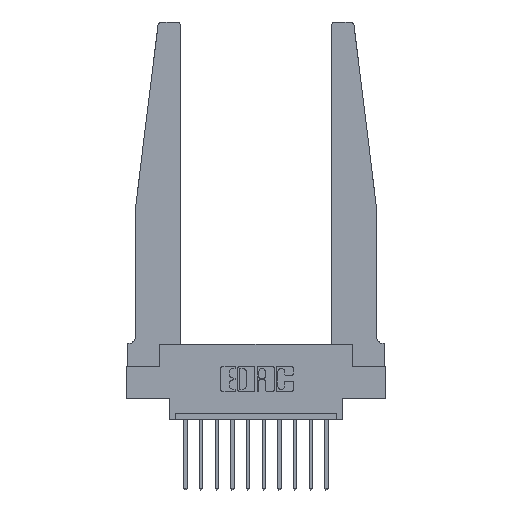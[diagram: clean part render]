
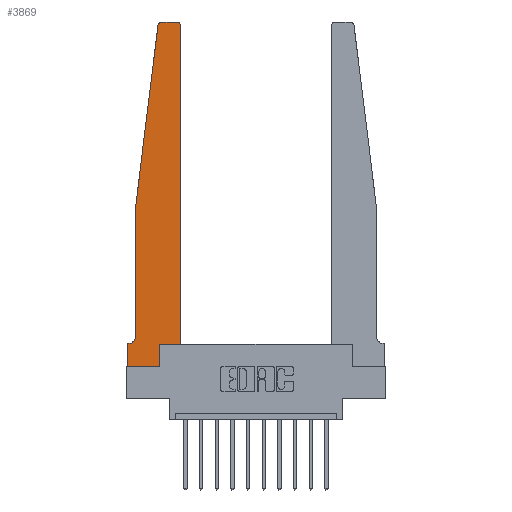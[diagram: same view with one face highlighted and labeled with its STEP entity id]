
A CAD part, top view. The second image highlights one B-rep face of the part: STEP entity #3869.
In plain terms, the highlighted planar face has unit normal (0, 0, 1).
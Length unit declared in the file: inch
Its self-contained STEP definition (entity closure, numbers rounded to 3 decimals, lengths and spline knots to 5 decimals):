
#71 = VECTOR ( 'NONE', #14322, 39.37008 ) ;
#1012 = VECTOR ( 'NONE', #14533, 39.37008 ) ;
#1158 = VERTEX_POINT ( 'NONE', #6319 ) ;
#1197 = ORIENTED_EDGE ( 'NONE', *, *, #5497, .T. ) ;
#1796 = CIRCLE ( 'NONE', #9764, 0.05 ) ;
#1976 = CARTESIAN_POINT ( 'NONE',  ( 0.2605, 0., 0.37 ) ) ;
#2045 = ORIENTED_EDGE ( 'NONE', *, *, #12021, .T. ) ;
#2255 = ORIENTED_EDGE ( 'NONE', *, *, #13639, .T. ) ;
#2366 = VERTEX_POINT ( 'NONE', #6105 ) ;
#2495 = VECTOR ( 'NONE', #3002, 39.37008 ) ;
#2706 = DIRECTION ( 'NONE',  ( 0., 0., 1. ) ) ;
#2829 = CARTESIAN_POINT ( 'NONE',  ( 0.25, 2.75, 0.37 ) ) ;
#2852 = CARTESIAN_POINT ( 'NONE',  ( 0.24675, 2.72367, 0.37 ) ) ;
#2860 = CARTESIAN_POINT ( 'NONE',  ( 0., 0., 0.37 ) ) ;
#2919 = EDGE_CURVE ( 'NONE', #6110, #9453, #13456, .T. ) ;
#2981 = CARTESIAN_POINT ( 'NONE',  ( 0.065, 1.25, 0.37 ) ) ;
#3002 = DIRECTION ( 'NONE',  ( 1., 0., 0. ) ) ;
#3043 = VECTOR ( 'NONE', #7891, 39.37008 ) ;
#3121 = FACE_OUTER_BOUND ( 'NONE', #15692, .T. ) ;
#3164 = CARTESIAN_POINT ( 'NONE',  ( 0.425, 0.18, 0.37 ) ) ;
#3613 = CARTESIAN_POINT ( 'NONE',  ( 0.27653, 2.75, 0.37 ) ) ;
#3869 = ADVANCED_FACE ( 'NONE', ( #3121 ), #15094, .T. ) ;
#4030 = DIRECTION ( 'NONE',  ( 0., 0., -1. ) ) ;
#4050 = EDGE_CURVE ( 'NONE', #10909, #1158, #6013, .T. ) ;
#4163 = DIRECTION ( 'NONE',  ( 1., 0., 0. ) ) ;
#4187 = LINE ( 'NONE', #2981, #3043 ) ;
#4429 = CARTESIAN_POINT ( 'NONE',  ( 0.425, 0.18, 0.37 ) ) ;
#4906 = ORIENTED_EDGE ( 'NONE', *, *, #12442, .T. ) ;
#4999 = CARTESIAN_POINT ( 'NONE',  ( 0.015, 0.2375, 0.37 ) ) ;
#5060 = VECTOR ( 'NONE', #11348, 39.37008 ) ;
#5497 = EDGE_CURVE ( 'NONE', #6813, #14636, #7718, .T. ) ;
#5702 = CARTESIAN_POINT ( 'NONE',  ( 0.065, 0.1875, 0.37 ) ) ;
#5705 = ORIENTED_EDGE ( 'NONE', *, *, #7953, .T. ) ;
#6013 = LINE ( 'NONE', #15486, #15292 ) ;
#6105 = CARTESIAN_POINT ( 'NONE',  ( 0.2605, 0.18, 0.37 ) ) ;
#6110 = VERTEX_POINT ( 'NONE', #8705 ) ;
#6305 = EDGE_CURVE ( 'NONE', #11668, #6110, #15426, .T. ) ;
#6319 = CARTESIAN_POINT ( 'NONE',  ( 0.065, 1.25, 0.37 ) ) ;
#6813 = VERTEX_POINT ( 'NONE', #2860 ) ;
#7058 = ORIENTED_EDGE ( 'NONE', *, *, #4050, .T. ) ;
#7499 = EDGE_CURVE ( 'NONE', #1158, #8719, #4187, .T. ) ;
#7537 = ORIENTED_EDGE ( 'NONE', *, *, #8444, .T. ) ;
#7700 = VERTEX_POINT ( 'NONE', #3613 ) ;
#7718 = LINE ( 'NONE', #14945, #5060 ) ;
#7891 = DIRECTION ( 'NONE',  ( 0., -1., 0. ) ) ;
#7933 = CIRCLE ( 'NONE', #11028, 0.03 ) ;
#7953 = EDGE_CURVE ( 'NONE', #9006, #15845, #10551, .T. ) ;
#8186 = CARTESIAN_POINT ( 'NONE',  ( 0.425, 0.18, 0.37 ) ) ;
#8212 = CARTESIAN_POINT ( 'NONE',  ( 0.065, 0.2375, 0.37 ) ) ;
#8260 = DIRECTION ( 'NONE',  ( -0.122, -0.992, 0. ) ) ;
#8275 = CARTESIAN_POINT ( 'NONE',  ( 0., 0., 0.37 ) ) ;
#8371 = LINE ( 'NONE', #15761, #12905 ) ;
#8444 = EDGE_CURVE ( 'NONE', #8719, #9006, #1796, .T. ) ;
#8705 = CARTESIAN_POINT ( 'NONE',  ( 0.425, 2.72, 0.37 ) ) ;
#8719 = VERTEX_POINT ( 'NONE', #8212 ) ;
#8927 = LINE ( 'NONE', #2829, #71 ) ;
#8940 = DIRECTION ( 'NONE',  ( -1., 0., 0. ) ) ;
#8989 = CARTESIAN_POINT ( 'NONE',  ( 0.395, 2.75, 0.37 ) ) ;
#9006 = VERTEX_POINT ( 'NONE', #14004 ) ;
#9335 = DIRECTION ( 'NONE',  ( 0., 1., 0. ) ) ;
#9358 = LINE ( 'NONE', #3164, #2495 ) ;
#9453 = VERTEX_POINT ( 'NONE', #8989 ) ;
#9570 = VECTOR ( 'NONE', #15505, 39.37008 ) ;
#9764 = AXIS2_PLACEMENT_3D ( 'NONE', #4999, #4030, #8940 ) ;
#10368 = DIRECTION ( 'NONE',  ( 0., 0., 1. ) ) ;
#10551 = LINE ( 'NONE', #5702, #1012 ) ;
#10583 = DIRECTION ( 'NONE',  ( 0., 1., 0. ) ) ;
#10752 = ORIENTED_EDGE ( 'NONE', *, *, #2919, .T. ) ;
#10830 = ORIENTED_EDGE ( 'NONE', *, *, #11289, .T. ) ;
#10873 = DIRECTION ( 'NONE',  ( 1., 0., 0. ) ) ;
#10909 = VERTEX_POINT ( 'NONE', #2852 ) ;
#11028 = AXIS2_PLACEMENT_3D ( 'NONE', #13051, #11862, #10873 ) ;
#11136 = AXIS2_PLACEMENT_3D ( 'NONE', #13734, #2706, #14682 ) ;
#11289 = EDGE_CURVE ( 'NONE', #9453, #7700, #8927, .T. ) ;
#11348 = DIRECTION ( 'NONE',  ( 1., 0., 0. ) ) ;
#11579 = CARTESIAN_POINT ( 'NONE',  ( 0., 0.1875, 0.37 ) ) ;
#11668 = VERTEX_POINT ( 'NONE', #8186 ) ;
#11862 = DIRECTION ( 'NONE',  ( 0., 0., 1. ) ) ;
#12021 = EDGE_CURVE ( 'NONE', #14636, #2366, #8371, .T. ) ;
#12207 = AXIS2_PLACEMENT_3D ( 'NONE', #14069, #10368, #4163 ) ;
#12442 = EDGE_CURVE ( 'NONE', #15845, #6813, #13191, .T. ) ;
#12905 = VECTOR ( 'NONE', #10583, 39.37008 ) ;
#12959 = ORIENTED_EDGE ( 'NONE', *, *, #6305, .T. ) ;
#13051 = CARTESIAN_POINT ( 'NONE',  ( 0.27653, 2.72, 0.37 ) ) ;
#13191 = LINE ( 'NONE', #8275, #9570 ) ;
#13228 = ORIENTED_EDGE ( 'NONE', *, *, #15130, .T. ) ;
#13456 = CIRCLE ( 'NONE', #11136, 0.03 ) ;
#13562 = VECTOR ( 'NONE', #9335, 39.37008 ) ;
#13639 = EDGE_CURVE ( 'NONE', #2366, #11668, #9358, .T. ) ;
#13734 = CARTESIAN_POINT ( 'NONE',  ( 0.395, 2.72, 0.37 ) ) ;
#14004 = CARTESIAN_POINT ( 'NONE',  ( 0.015, 0.1875, 0.37 ) ) ;
#14069 = CARTESIAN_POINT ( 'NONE',  ( 0., 0.1875, 0.37 ) ) ;
#14322 = DIRECTION ( 'NONE',  ( -1., 0., 0. ) ) ;
#14533 = DIRECTION ( 'NONE',  ( -1., 0., 0. ) ) ;
#14636 = VERTEX_POINT ( 'NONE', #1976 ) ;
#14682 = DIRECTION ( 'NONE',  ( 1., 0., 0. ) ) ;
#14945 = CARTESIAN_POINT ( 'NONE',  ( 0., 0., 0.37 ) ) ;
#15094 = PLANE ( 'NONE',  #12207 ) ;
#15130 = EDGE_CURVE ( 'NONE', #7700, #10909, #7933, .T. ) ;
#15292 = VECTOR ( 'NONE', #8260, 39.37008 ) ;
#15426 = LINE ( 'NONE', #4429, #13562 ) ;
#15486 = CARTESIAN_POINT ( 'NONE',  ( 0.065, 1.25, 0.37 ) ) ;
#15505 = DIRECTION ( 'NONE',  ( 0., -1., 0. ) ) ;
#15692 = EDGE_LOOP ( 'NONE', ( #10830, #13228, #7058, #15810, #7537, #5705, #4906, #1197, #2045, #2255, #12959, #10752 ) ) ;
#15761 = CARTESIAN_POINT ( 'NONE',  ( 0.2605, 0.18, 0.37 ) ) ;
#15810 = ORIENTED_EDGE ( 'NONE', *, *, #7499, .T. ) ;
#15845 = VERTEX_POINT ( 'NONE', #11579 ) ;
